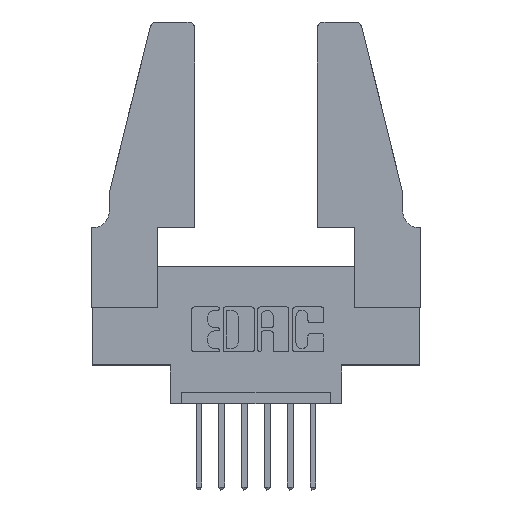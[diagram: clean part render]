
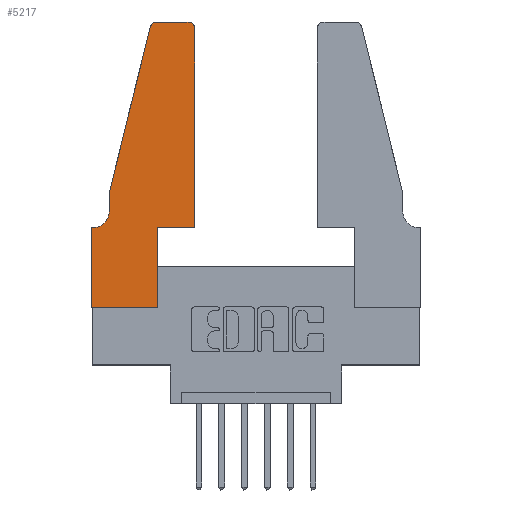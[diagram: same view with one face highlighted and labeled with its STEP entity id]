
A CAD part, top view. The second image highlights one B-rep face of the part: STEP entity #5217.
In plain terms, the highlighted planar face has unit normal (0, 0, 1).
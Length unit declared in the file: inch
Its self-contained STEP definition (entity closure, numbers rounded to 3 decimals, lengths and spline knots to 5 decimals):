
#160 = VECTOR ( 'NONE', #11401, 39.37008 ) ;
#229 = VERTEX_POINT ( 'NONE', #4150 ) ;
#519 = CARTESIAN_POINT ( 'NONE',  ( 0.2865, 0.35, 0.37 ) ) ;
#672 = LINE ( 'NONE', #2889, #815 ) ;
#815 = VECTOR ( 'NONE', #6458, 39.37008 ) ;
#1236 = EDGE_CURVE ( 'NONE', #4798, #3432, #10310, .T. ) ;
#1459 = EDGE_CURVE ( 'NONE', #6349, #10109, #5492, .T. ) ;
#1571 = ORIENTED_EDGE ( 'NONE', *, *, #9213, .T. ) ;
#1600 = DIRECTION ( 'NONE',  ( 1., 0., 0. ) ) ;
#1646 = CARTESIAN_POINT ( 'NONE',  ( 0.4205, 1.22, 0.37 ) ) ;
#1648 = LINE ( 'NONE', #4920, #10392 ) ;
#1802 = CARTESIAN_POINT ( 'NONE',  ( 0.0755, 0.35, 0.37 ) ) ;
#2334 = CARTESIAN_POINT ( 'NONE',  ( 0.25487, 1.22718, 0.37 ) ) ;
#2374 = ORIENTED_EDGE ( 'NONE', *, *, #1459, .T. ) ;
#2545 = ORIENTED_EDGE ( 'NONE', *, *, #3118, .T. ) ;
#2889 = CARTESIAN_POINT ( 'NONE',  ( 0.4505, 0.35, 0.37 ) ) ;
#3118 = EDGE_CURVE ( 'NONE', #3432, #10035, #11098, .T. ) ;
#3165 = ORIENTED_EDGE ( 'NONE', *, *, #10628, .T. ) ;
#3178 = PLANE ( 'NONE',  #6577 ) ;
#3312 = AXIS2_PLACEMENT_3D ( 'NONE', #6035, #10591, #8969 ) ;
#3432 = VERTEX_POINT ( 'NONE', #5770 ) ;
#3433 = CARTESIAN_POINT ( 'NONE',  ( 0.4505, 0.35, 0.37 ) ) ;
#3459 = VECTOR ( 'NONE', #6022, 39.37008 ) ;
#3484 = ORIENTED_EDGE ( 'NONE', *, *, #4234, .T. ) ;
#3513 = VECTOR ( 'NONE', #9755, 39.37008 ) ;
#3616 = EDGE_CURVE ( 'NONE', #9901, #3986, #4892, .T. ) ;
#3704 = CARTESIAN_POINT ( 'NONE',  ( 0.4205, 1.25, 0.37 ) ) ;
#3740 = DIRECTION ( 'NONE',  ( 0., -1., 0. ) ) ;
#3755 = LINE ( 'NONE', #3999, #5323 ) ;
#3986 = VERTEX_POINT ( 'NONE', #10113 ) ;
#3999 = CARTESIAN_POINT ( 'NONE',  ( 0.2605, 1.25, 0.37 ) ) ;
#4137 = CARTESIAN_POINT ( 'NONE',  ( 0., 0.35, 0.37 ) ) ;
#4145 = CARTESIAN_POINT ( 'NONE',  ( 0.284, 1.25, 0.37 ) ) ;
#4150 = CARTESIAN_POINT ( 'NONE',  ( 0.4505, 1.22, 0.37 ) ) ;
#4217 = CARTESIAN_POINT ( 'NONE',  ( 0.0755, 0.5, 0.37 ) ) ;
#4234 = EDGE_CURVE ( 'NONE', #6449, #6349, #9667, .T. ) ;
#4381 = CARTESIAN_POINT ( 'NONE',  ( 0.0755, 0.5, 0.37 ) ) ;
#4423 = ORIENTED_EDGE ( 'NONE', *, *, #1236, .T. ) ;
#4448 = CARTESIAN_POINT ( 'NONE',  ( 0.0755, 0.42, 0.37 ) ) ;
#4798 = VERTEX_POINT ( 'NONE', #8799 ) ;
#4850 = DIRECTION ( 'NONE',  ( -1., 0., 0. ) ) ;
#4892 = CIRCLE ( 'NONE', #3312, 0.07 ) ;
#4920 = CARTESIAN_POINT ( 'NONE',  ( 0., 0., 0.37 ) ) ;
#5217 = ADVANCED_FACE ( 'NONE', ( #5705 ), #3178, .T. ) ;
#5323 = VECTOR ( 'NONE', #4850, 39.37008 ) ;
#5492 = LINE ( 'NONE', #4217, #3513 ) ;
#5705 = FACE_OUTER_BOUND ( 'NONE', #9044, .T. ) ;
#5770 = CARTESIAN_POINT ( 'NONE',  ( 0.2865, 0.35, 0.37 ) ) ;
#6012 = VECTOR ( 'NONE', #3740, 39.37008 ) ;
#6022 = DIRECTION ( 'NONE',  ( 1., 0., 0. ) ) ;
#6035 = CARTESIAN_POINT ( 'NONE',  ( 0.0055, 0.42, 0.37 ) ) ;
#6142 = ORIENTED_EDGE ( 'NONE', *, *, #10443, .T. ) ;
#6167 = DIRECTION ( 'NONE',  ( 0., 0., 1. ) ) ;
#6349 = VERTEX_POINT ( 'NONE', #2334 ) ;
#6393 = CARTESIAN_POINT ( 'NONE',  ( 0., 0.35, 0.37 ) ) ;
#6449 = VERTEX_POINT ( 'NONE', #4145 ) ;
#6458 = DIRECTION ( 'NONE',  ( 0., 1., 0. ) ) ;
#6462 = DIRECTION ( 'NONE',  ( -1., 0., 0. ) ) ;
#6569 = VECTOR ( 'NONE', #11055, 39.37008 ) ;
#6577 = AXIS2_PLACEMENT_3D ( 'NONE', #4137, #9596, #7733 ) ;
#7281 = ORIENTED_EDGE ( 'NONE', *, *, #3616, .T. ) ;
#7418 = ORIENTED_EDGE ( 'NONE', *, *, #9923, .T. ) ;
#7443 = CARTESIAN_POINT ( 'NONE',  ( 0.4505, 0.35, 0.37 ) ) ;
#7673 = AXIS2_PLACEMENT_3D ( 'NONE', #1646, #6167, #11595 ) ;
#7733 = DIRECTION ( 'NONE',  ( 1., 0., 0. ) ) ;
#7909 = CARTESIAN_POINT ( 'NONE',  ( 0.284, 1.22, 0.37 ) ) ;
#7993 = LINE ( 'NONE', #1802, #10822 ) ;
#8137 = LINE ( 'NONE', #10573, #3459 ) ;
#8692 = DIRECTION ( 'NONE',  ( 0., 0., 1. ) ) ;
#8753 = ORIENTED_EDGE ( 'NONE', *, *, #9881, .T. ) ;
#8799 = CARTESIAN_POINT ( 'NONE',  ( 0.2865, 0., 0.37 ) ) ;
#8969 = DIRECTION ( 'NONE',  ( -1., 0., 0. ) ) ;
#8988 = CIRCLE ( 'NONE', #7673, 0.03 ) ;
#9044 = EDGE_LOOP ( 'NONE', ( #10172, #3484, #2374, #6142, #7281, #7418, #3165, #8753, #4423, #2545, #1571, #10298 ) ) ;
#9213 = EDGE_CURVE ( 'NONE', #10035, #229, #672, .T. ) ;
#9596 = DIRECTION ( 'NONE',  ( 0., 0., 1. ) ) ;
#9638 = EDGE_CURVE ( 'NONE', #229, #11630, #8988, .T. ) ;
#9667 = CIRCLE ( 'NONE', #10888, 0.03 ) ;
#9755 = DIRECTION ( 'NONE',  ( -0.239, -0.971, 0. ) ) ;
#9881 = EDGE_CURVE ( 'NONE', #11021, #4798, #8137, .T. ) ;
#9901 = VERTEX_POINT ( 'NONE', #4448 ) ;
#9923 = EDGE_CURVE ( 'NONE', #3986, #11600, #7993, .T. ) ;
#10035 = VERTEX_POINT ( 'NONE', #3433 ) ;
#10109 = VERTEX_POINT ( 'NONE', #11297 ) ;
#10113 = CARTESIAN_POINT ( 'NONE',  ( 0.0055, 0.35, 0.37 ) ) ;
#10172 = ORIENTED_EDGE ( 'NONE', *, *, #10736, .T. ) ;
#10264 = LINE ( 'NONE', #4381, #6012 ) ;
#10298 = ORIENTED_EDGE ( 'NONE', *, *, #9638, .T. ) ;
#10310 = LINE ( 'NONE', #519, #160 ) ;
#10392 = VECTOR ( 'NONE', #11225, 39.37008 ) ;
#10443 = EDGE_CURVE ( 'NONE', #10109, #9901, #10264, .T. ) ;
#10573 = CARTESIAN_POINT ( 'NONE',  ( 0., 0., 0.37 ) ) ;
#10591 = DIRECTION ( 'NONE',  ( 0., 0., -1. ) ) ;
#10628 = EDGE_CURVE ( 'NONE', #11600, #11021, #1648, .T. ) ;
#10736 = EDGE_CURVE ( 'NONE', #11630, #6449, #3755, .T. ) ;
#10822 = VECTOR ( 'NONE', #6462, 39.37008 ) ;
#10888 = AXIS2_PLACEMENT_3D ( 'NONE', #7909, #8692, #1600 ) ;
#11021 = VERTEX_POINT ( 'NONE', #11474 ) ;
#11055 = DIRECTION ( 'NONE',  ( 1., 0., 0. ) ) ;
#11098 = LINE ( 'NONE', #7443, #6569 ) ;
#11225 = DIRECTION ( 'NONE',  ( 0., -1., 0. ) ) ;
#11297 = CARTESIAN_POINT ( 'NONE',  ( 0.0755, 0.5, 0.37 ) ) ;
#11401 = DIRECTION ( 'NONE',  ( 0., 1., 0. ) ) ;
#11474 = CARTESIAN_POINT ( 'NONE',  ( 0., 0., 0.37 ) ) ;
#11595 = DIRECTION ( 'NONE',  ( 1., 0., 0. ) ) ;
#11600 = VERTEX_POINT ( 'NONE', #6393 ) ;
#11630 = VERTEX_POINT ( 'NONE', #3704 ) ;
